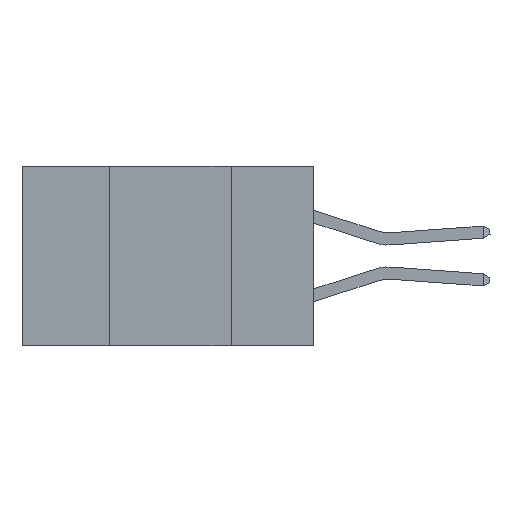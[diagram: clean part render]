
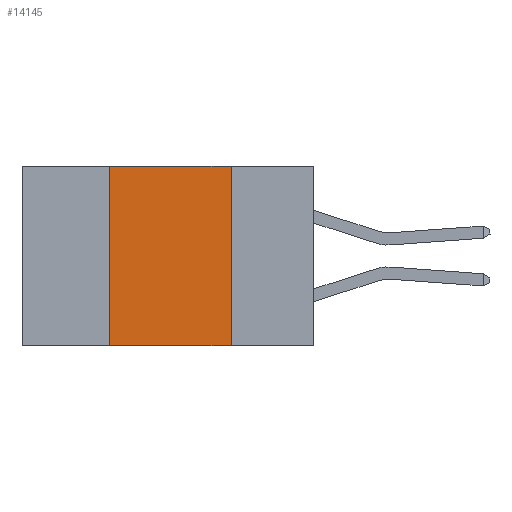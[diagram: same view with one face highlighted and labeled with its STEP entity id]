
A CAD part, left-side view. The second image highlights one B-rep face of the part: STEP entity #14145.
In plain terms, the highlighted planar face has unit normal (-1, 0, 0).
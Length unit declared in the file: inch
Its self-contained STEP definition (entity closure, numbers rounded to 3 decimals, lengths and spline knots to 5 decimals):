
#722 = VERTEX_POINT ( 'NONE', #4257 ) ;
#935 = VERTEX_POINT ( 'NONE', #5749 ) ;
#954 = CARTESIAN_POINT ( 'NONE',  ( 0., 0.42, -0.37 ) ) ;
#1304 = CARTESIAN_POINT ( 'NONE',  ( 0., 0.17, 0. ) ) ;
#2425 = ORIENTED_EDGE ( 'NONE', *, *, #7281, .F. ) ;
#4191 = DIRECTION ( 'NONE',  ( 0., 0., -1. ) ) ;
#4257 = CARTESIAN_POINT ( 'NONE',  ( 0., 0.42, 0. ) ) ;
#4345 = VECTOR ( 'NONE', #4191, 39.37008 ) ;
#4756 = PLANE ( 'NONE',  #15026 ) ;
#4947 = EDGE_LOOP ( 'NONE', ( #2425, #6878, #13354, #18327 ) ) ;
#5523 = CARTESIAN_POINT ( 'NONE',  ( 0., 0.42, 0. ) ) ;
#5749 = CARTESIAN_POINT ( 'NONE',  ( 0., 0.17, -0.37 ) ) ;
#6495 = LINE ( 'NONE', #5523, #14032 ) ;
#6878 = ORIENTED_EDGE ( 'NONE', *, *, #16287, .F. ) ;
#7189 = VERTEX_POINT ( 'NONE', #954 ) ;
#7281 = EDGE_CURVE ( 'NONE', #13421, #935, #13750, .T. ) ;
#7750 = CARTESIAN_POINT ( 'NONE',  ( 0., 0.6, 0. ) ) ;
#8726 = DIRECTION ( 'NONE',  ( 0., -1., 0. ) ) ;
#8937 = CARTESIAN_POINT ( 'NONE',  ( 0., 0.6, -0.37 ) ) ;
#9253 = DIRECTION ( 'NONE',  ( 0., 0., -1. ) ) ;
#9262 = FACE_OUTER_BOUND ( 'NONE', #4947, .T. ) ;
#10832 = EDGE_CURVE ( 'NONE', #7189, #722, #6495, .T. ) ;
#12039 = VECTOR ( 'NONE', #19404, 39.37008 ) ;
#12522 = LINE ( 'NONE', #8937, #12039 ) ;
#13354 = ORIENTED_EDGE ( 'NONE', *, *, #10832, .F. ) ;
#13421 = VERTEX_POINT ( 'NONE', #1304 ) ;
#13452 = VECTOR ( 'NONE', #8726, 39.37008 ) ;
#13750 = LINE ( 'NONE', #14668, #4345 ) ;
#14032 = VECTOR ( 'NONE', #14521, 39.37008 ) ;
#14145 = ADVANCED_FACE ( 'NONE', ( #9262 ), #4756, .F. ) ;
#14521 = DIRECTION ( 'NONE',  ( 0., 0., 1. ) ) ;
#14668 = CARTESIAN_POINT ( 'NONE',  ( 0., 0.17, 0. ) ) ;
#15026 = AXIS2_PLACEMENT_3D ( 'NONE', #7750, #18277, #9253 ) ;
#16287 = EDGE_CURVE ( 'NONE', #722, #13421, #17468, .T. ) ;
#16387 = EDGE_CURVE ( 'NONE', #7189, #935, #12522, .T. ) ;
#17468 = LINE ( 'NONE', #17750, #13452 ) ;
#17750 = CARTESIAN_POINT ( 'NONE',  ( 0., 0.6, 0. ) ) ;
#18277 = DIRECTION ( 'NONE',  ( 1., 0., 0. ) ) ;
#18327 = ORIENTED_EDGE ( 'NONE', *, *, #16387, .T. ) ;
#19404 = DIRECTION ( 'NONE',  ( 0., -1., 0. ) ) ;
